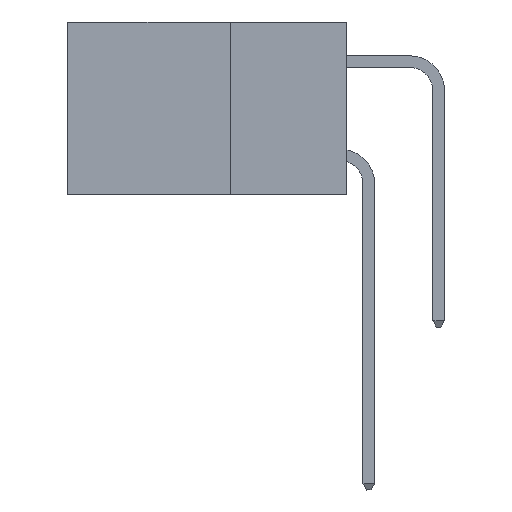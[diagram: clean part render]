
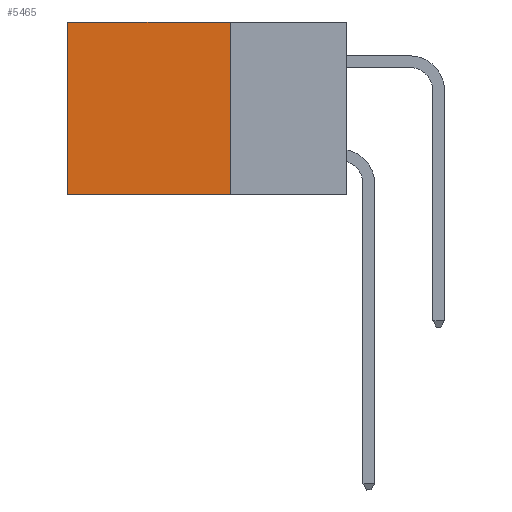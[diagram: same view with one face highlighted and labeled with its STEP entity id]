
A CAD part, left-side view. The second image highlights one B-rep face of the part: STEP entity #5465.
In plain terms, the highlighted planar face has unit normal (-1, 0, 0).
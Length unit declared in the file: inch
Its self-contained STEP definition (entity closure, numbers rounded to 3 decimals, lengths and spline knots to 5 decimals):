
#647 = CARTESIAN_POINT ( 'NONE',  ( 0.2875, 0.25, -0.37 ) ) ;
#1226 = PLANE ( 'NONE',  #16014 ) ;
#1360 = CARTESIAN_POINT ( 'NONE',  ( 0.2875, 0.25, 0. ) ) ;
#1759 = ORIENTED_EDGE ( 'NONE', *, *, #15094, .T. ) ;
#2446 = LINE ( 'NONE', #5148, #5321 ) ;
#3832 = EDGE_CURVE ( 'NONE', #12047, #7369, #10911, .T. ) ;
#4519 = CARTESIAN_POINT ( 'NONE',  ( 0.2875, 0.25, -0.37 ) ) ;
#4892 = FACE_OUTER_BOUND ( 'NONE', #5875, .T. ) ;
#5065 = VERTEX_POINT ( 'NONE', #14356 ) ;
#5148 = CARTESIAN_POINT ( 'NONE',  ( 0.2875, 0.25, 0. ) ) ;
#5321 = VECTOR ( 'NONE', #11744, 39.37008 ) ;
#5465 = ADVANCED_FACE ( 'NONE', ( #4892 ), #1226, .F. ) ;
#5817 = CARTESIAN_POINT ( 'NONE',  ( 0.2875, 0.25, 0. ) ) ;
#5875 = EDGE_LOOP ( 'NONE', ( #1759, #16189, #15389, #5956 ) ) ;
#5956 = ORIENTED_EDGE ( 'NONE', *, *, #13683, .T. ) ;
#6473 = EDGE_CURVE ( 'NONE', #7369, #5065, #9860, .T. ) ;
#6935 = CARTESIAN_POINT ( 'NONE',  ( 0.2875, 0.6, 0. ) ) ;
#7369 = VERTEX_POINT ( 'NONE', #4519 ) ;
#7441 = VERTEX_POINT ( 'NONE', #12254 ) ;
#9801 = DIRECTION ( 'NONE',  ( 0., 1., 0. ) ) ;
#9860 = LINE ( 'NONE', #647, #12986 ) ;
#9877 = DIRECTION ( 'NONE',  ( 0., 0., -1. ) ) ;
#10911 = LINE ( 'NONE', #1360, #12391 ) ;
#11744 = DIRECTION ( 'NONE',  ( 0., 1., 0. ) ) ;
#11948 = CARTESIAN_POINT ( 'NONE',  ( 0.2875, 0.25, 0. ) ) ;
#12047 = VERTEX_POINT ( 'NONE', #11948 ) ;
#12254 = CARTESIAN_POINT ( 'NONE',  ( 0.2875, 0.6, 0. ) ) ;
#12277 = VECTOR ( 'NONE', #12459, 39.37008 ) ;
#12391 = VECTOR ( 'NONE', #9877, 39.37008 ) ;
#12459 = DIRECTION ( 'NONE',  ( 0., 0., -1. ) ) ;
#12986 = VECTOR ( 'NONE', #9801, 39.37008 ) ;
#13683 = EDGE_CURVE ( 'NONE', #12047, #7441, #2446, .T. ) ;
#14308 = LINE ( 'NONE', #6935, #12277 ) ;
#14356 = CARTESIAN_POINT ( 'NONE',  ( 0.2875, 0.6, -0.37 ) ) ;
#14395 = DIRECTION ( 'NONE',  ( 1., 0., 0. ) ) ;
#15094 = EDGE_CURVE ( 'NONE', #7441, #5065, #14308, .T. ) ;
#15389 = ORIENTED_EDGE ( 'NONE', *, *, #3832, .F. ) ;
#15643 = DIRECTION ( 'NONE',  ( 0., 0., -1. ) ) ;
#16014 = AXIS2_PLACEMENT_3D ( 'NONE', #5817, #14395, #15643 ) ;
#16189 = ORIENTED_EDGE ( 'NONE', *, *, #6473, .F. ) ;
